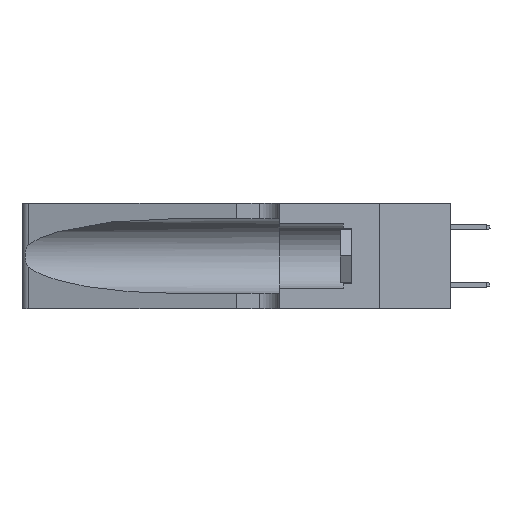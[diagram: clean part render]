
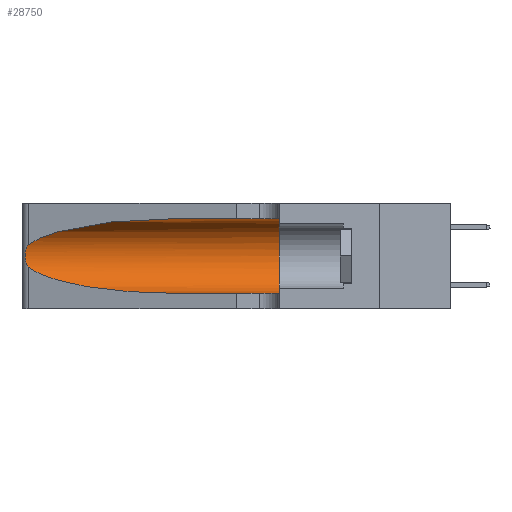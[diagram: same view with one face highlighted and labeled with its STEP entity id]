
A CAD part, left-side view. The second image highlights one B-rep face of the part: STEP entity #28750.
In plain terms, the highlighted cylindrical face has radius 3.308 mm (diameter 6.617 mm), a partial arc.
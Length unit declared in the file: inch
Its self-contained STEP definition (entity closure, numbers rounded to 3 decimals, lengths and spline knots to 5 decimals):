
#159 = CARTESIAN_POINT ( 'NONE',  ( 0.1305, 0.72297, 0.31525 ) ) ;
#1468 = CARTESIAN_POINT ( 'NONE',  ( 0.1305, 0.35, 0.05475 ) ) ;
#1673 =( BOUNDED_CURVE ( )  B_SPLINE_CURVE ( 3, ( #21379, #14976, #24795, #7917 ),
 .UNSPECIFIED., .F., .F. ) 
 B_SPLINE_CURVE_WITH_KNOTS ( ( 4, 4 ),
 ( 3.44316, 4.71239 ),
 .UNSPECIFIED. ) 
 CURVE ( )  GEOMETRIC_REPRESENTATION_ITEM ( )  RATIONAL_B_SPLINE_CURVE ( ( 1., 0.87, 0.87, 1. ) ) 
 REPRESENTATION_ITEM ( '' )  );
#1674 = CARTESIAN_POINT ( 'NONE',  ( 0.26017, 1.23833, 0.17102 ) ) ;
#2676 = DIRECTION ( 'NONE',  ( 0., 1., 0. ) ) ;
#3798 = ORIENTED_EDGE ( 'NONE', *, *, #43177, .F. ) ;
#5099 = CARTESIAN_POINT ( 'NONE',  ( 0.25854, 1.2359, 0.20912 ) ) ;
#5422 = DIRECTION ( 'NONE',  ( 0., 0., 1. ) ) ;
#5490 = CARTESIAN_POINT ( 'NONE',  ( 0.1305, 1.61858, 0.31525 ) ) ;
#6942 = CARTESIAN_POINT ( 'NONE',  ( 0.1305, 1.61858, 0.05475 ) ) ;
#7854 = VERTEX_POINT ( 'NONE', #25492 ) ;
#7909 = CARTESIAN_POINT ( 'NONE',  ( 0.2373, 1.15595, 0.28018 ) ) ;
#7917 = CARTESIAN_POINT ( 'NONE',  ( 0.1305, 0.72297, 0.05475 ) ) ;
#8724 = CARTESIAN_POINT ( 'NONE',  ( 0.26075, 1.23896, 0.19203 ) ) ;
#9350 = DIRECTION ( 'NONE',  ( 0., -1., 0. ) ) ;
#12374 = CARTESIAN_POINT ( 'NONE',  ( 0.25487, 1.22718, 0.22369 ) ) ;
#12408 = VERTEX_POINT ( 'NONE', #16601 ) ;
#14802 = AXIS2_PLACEMENT_3D ( 'NONE', #33648, #19552, #16122 ) ;
#14976 = CARTESIAN_POINT ( 'NONE',  ( 0.2373, 1.15595, 0.08982 ) ) ;
#15571 = CARTESIAN_POINT ( 'NONE',  ( 0.25856, 1.23593, 0.16098 ) ) ;
#15740 = VECTOR ( 'NONE', #24506, 39.37008 ) ;
#16006 = CARTESIAN_POINT ( 'NONE',  ( 0.25555, 1.22993, 0.14849 ) ) ;
#16122 = DIRECTION ( 'NONE',  ( 0., 0., -1. ) ) ;
#16601 = CARTESIAN_POINT ( 'NONE',  ( 0.1305, 0.72297, 0.05475 ) ) ;
#17432 = VERTEX_POINT ( 'NONE', #25347 ) ;
#18323 = EDGE_CURVE ( 'NONE', #7854, #19365, #26176, .T. ) ;
#19365 = VERTEX_POINT ( 'NONE', #23216 ) ;
#19552 = DIRECTION ( 'NONE',  ( 0., -1., 0. ) ) ;
#21379 = CARTESIAN_POINT ( 'NONE',  ( 0.25487, 1.22718, 0.14631 ) ) ;
#22643 = CARTESIAN_POINT ( 'NONE',  ( 0.25789, 1.23486, 0.15765 ) ) ;
#23216 = CARTESIAN_POINT ( 'NONE',  ( 0.25487, 1.22718, 0.22369 ) ) ;
#23345 = ORIENTED_EDGE ( 'NONE', *, *, #33764, .T. ) ;
#24186 = EDGE_CURVE ( 'NONE', #42875, #12408, #1673, .T. ) ;
#24506 = DIRECTION ( 'NONE',  ( 0., -1., 0. ) ) ;
#24545 = CARTESIAN_POINT ( 'NONE',  ( 0.18966, 0.96281, 0.31525 ) ) ;
#24795 = CARTESIAN_POINT ( 'NONE',  ( 0.18966, 0.96281, 0.05475 ) ) ;
#25347 = CARTESIAN_POINT ( 'NONE',  ( 0.1305, 0.35, 0.31525 ) ) ;
#25492 = CARTESIAN_POINT ( 'NONE',  ( 0.1305, 0.72297, 0.31525 ) ) ;
#26176 =( BOUNDED_CURVE ( )  B_SPLINE_CURVE ( 3, ( #159, #24545, #7909, #38868 ),
 .UNSPECIFIED., .F., .F. ) 
 B_SPLINE_CURVE_WITH_KNOTS ( ( 4, 4 ),
 ( 1.5708, 2.84003 ),
 .UNSPECIFIED. ) 
 CURVE ( )  GEOMETRIC_REPRESENTATION_ITEM ( )  RATIONAL_B_SPLINE_CURVE ( ( 1., 0.87, 0.87, 1. ) ) 
 REPRESENTATION_ITEM ( '' )  );
#26280 = CARTESIAN_POINT ( 'NONE',  ( 0.25639, 1.23184, 0.21858 ) ) ;
#27066 = CYLINDRICAL_SURFACE ( 'NONE', #14802, 0.13025 ) ;
#28750 = ADVANCED_FACE ( 'NONE', ( #34322 ), #27066, .F. ) ;
#29451 = CARTESIAN_POINT ( 'NONE',  ( 0.25639, 1.23186, 0.15144 ) ) ;
#29862 = ORIENTED_EDGE ( 'NONE', *, *, #32024, .T. ) ;
#29892 = CARTESIAN_POINT ( 'NONE',  ( 0.25487, 1.22718, 0.14631 ) ) ;
#29995 = CARTESIAN_POINT ( 'NONE',  ( 0.1305, 0.35, 0.185 ) ) ;
#31454 = B_SPLINE_CURVE_WITH_KNOTS ( 'NONE', 3,
 ( #12374, #33091, #26280, #36281, #5099, #33314, #8724, #32871, #1674, #15571, #22643, #29451, #16006, #29892 ),
 .UNSPECIFIED., .F., .F.,
 ( 4, 2, 2, 2, 2, 2, 4 ),
 ( 0., 0.00027, 0.00053, 0.00107, 0.0016, 0.00187, 0.00214 ),
 .UNSPECIFIED. ) ;
#32024 = EDGE_CURVE ( 'NONE', #12408, #42511, #39062, .T. ) ;
#32871 = CARTESIAN_POINT ( 'NONE',  ( 0.26075, 1.23896, 0.178 ) ) ;
#33091 = CARTESIAN_POINT ( 'NONE',  ( 0.25555, 1.22994, 0.2215 ) ) ;
#33314 = CARTESIAN_POINT ( 'NONE',  ( 0.26018, 1.23835, 0.19895 ) ) ;
#33412 = AXIS2_PLACEMENT_3D ( 'NONE', #29995, #2676, #5422 ) ;
#33648 = CARTESIAN_POINT ( 'NONE',  ( 0.1305, 1.61858, 0.185 ) ) ;
#33764 = EDGE_CURVE ( 'NONE', #19365, #42875, #31454, .T. ) ;
#34322 = FACE_OUTER_BOUND ( 'NONE', #39395, .T. ) ;
#36281 = CARTESIAN_POINT ( 'NONE',  ( 0.25787, 1.23484, 0.2124 ) ) ;
#36667 = LINE ( 'NONE', #5490, #39611 ) ;
#37575 = EDGE_CURVE ( 'NONE', #17432, #42511, #42889, .T. ) ;
#38752 = CARTESIAN_POINT ( 'NONE',  ( 0.25487, 1.22718, 0.14631 ) ) ;
#38868 = CARTESIAN_POINT ( 'NONE',  ( 0.25487, 1.22718, 0.22369 ) ) ;
#39047 = ORIENTED_EDGE ( 'NONE', *, *, #37575, .F. ) ;
#39062 = LINE ( 'NONE', #6942, #15740 ) ;
#39395 = EDGE_LOOP ( 'NONE', ( #39928, #23345, #41139, #29862, #39047, #3798 ) ) ;
#39611 = VECTOR ( 'NONE', #9350, 39.37008 ) ;
#39928 = ORIENTED_EDGE ( 'NONE', *, *, #18323, .T. ) ;
#41139 = ORIENTED_EDGE ( 'NONE', *, *, #24186, .T. ) ;
#42511 = VERTEX_POINT ( 'NONE', #1468 ) ;
#42875 = VERTEX_POINT ( 'NONE', #38752 ) ;
#42889 = CIRCLE ( 'NONE', #33412, 0.13025 ) ;
#43177 = EDGE_CURVE ( 'NONE', #7854, #17432, #36667, .T. ) ;
